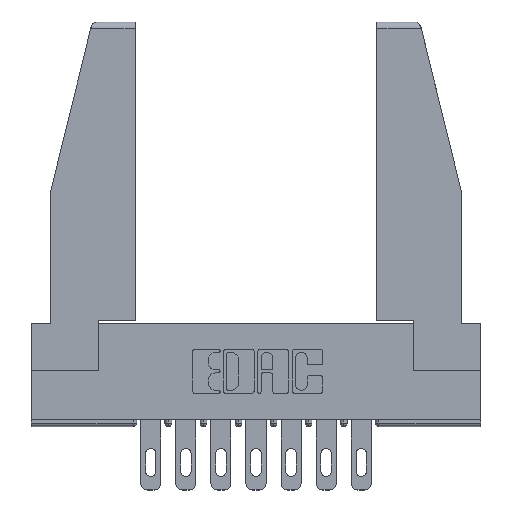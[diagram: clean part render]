
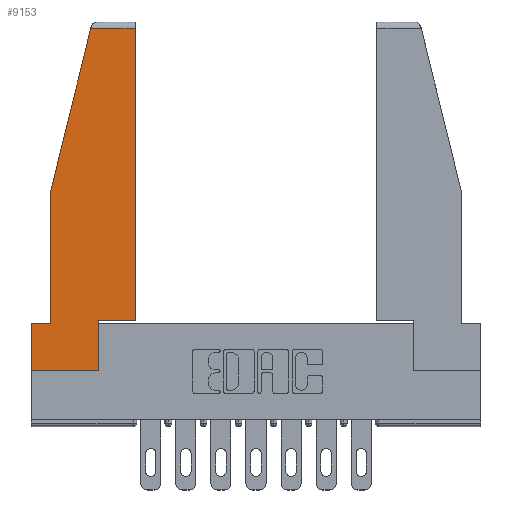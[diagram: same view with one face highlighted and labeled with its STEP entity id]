
A CAD part, top view. The second image highlights one B-rep face of the part: STEP entity #9153.
In plain terms, the highlighted planar face has unit normal (0, 0, 1).
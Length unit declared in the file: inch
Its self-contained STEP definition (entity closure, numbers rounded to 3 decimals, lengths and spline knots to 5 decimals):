
#136 = EDGE_CURVE ( 'NONE', #3867, #2991, #2911, .T. ) ;
#413 = LINE ( 'NONE', #6282, #13234 ) ;
#431 = LINE ( 'NONE', #12536, #7899 ) ;
#455 = VERTEX_POINT ( 'NONE', #8665 ) ;
#515 = DIRECTION ( 'NONE',  ( -1., 0., 0. ) ) ;
#610 = VECTOR ( 'NONE', #1914, 39.37008 ) ;
#940 = CARTESIAN_POINT ( 'NONE',  ( 0., 0.21, 0. ) ) ;
#1140 = ORIENTED_EDGE ( 'NONE', *, *, #8603, .T. ) ;
#1431 = DIRECTION ( 'NONE',  ( 0., 1., 0. ) ) ;
#1530 = ORIENTED_EDGE ( 'NONE', *, *, #7670, .T. ) ;
#1914 = DIRECTION ( 'NONE',  ( 0., 1., 0. ) ) ;
#2023 = LINE ( 'NONE', #5896, #12410 ) ;
#2159 = CARTESIAN_POINT ( 'NONE',  ( 0.086, 0.21, 0. ) ) ;
#2171 = VERTEX_POINT ( 'NONE', #7462 ) ;
#2279 = ORIENTED_EDGE ( 'NONE', *, *, #4471, .T. ) ;
#2459 = AXIS2_PLACEMENT_3D ( 'NONE', #3951, #11770, #9659 ) ;
#2619 = CARTESIAN_POINT ( 'NONE',  ( 0.297, 0., 0. ) ) ;
#2677 = CARTESIAN_POINT ( 'NONE',  ( 0.297, 0.223, 0. ) ) ;
#2857 = VERTEX_POINT ( 'NONE', #3028 ) ;
#2911 = LINE ( 'NONE', #6354, #7980 ) ;
#2991 = VERTEX_POINT ( 'NONE', #2159 ) ;
#3028 = CARTESIAN_POINT ( 'NONE',  ( 0., 0.21, 0. ) ) ;
#3124 = ORIENTED_EDGE ( 'NONE', *, *, #5001, .T. ) ;
#3164 = ORIENTED_EDGE ( 'NONE', *, *, #13414, .T. ) ;
#3232 = LINE ( 'NONE', #5779, #13629 ) ;
#3373 = CARTESIAN_POINT ( 'NONE',  ( 0.461, 1.52, 0. ) ) ;
#3582 = VERTEX_POINT ( 'NONE', #2677 ) ;
#3867 = VERTEX_POINT ( 'NONE', #7678 ) ;
#3951 = CARTESIAN_POINT ( 'NONE',  ( 0., 0., 0. ) ) ;
#4002 = CARTESIAN_POINT ( 'NONE',  ( 0.461, 0.223, 0. ) ) ;
#4132 = EDGE_LOOP ( 'NONE', ( #1140, #3124, #1530, #4251, #3164, #4920, #13564, #2279, #6168 ) ) ;
#4251 = ORIENTED_EDGE ( 'NONE', *, *, #136, .T. ) ;
#4471 = EDGE_CURVE ( 'NONE', #11924, #3582, #9983, .T. ) ;
#4920 = ORIENTED_EDGE ( 'NONE', *, *, #8428, .T. ) ;
#4953 = CARTESIAN_POINT ( 'NONE',  ( 0., 1.52, 0. ) ) ;
#5001 = EDGE_CURVE ( 'NONE', #6144, #9049, #10142, .T. ) ;
#5779 = CARTESIAN_POINT ( 'NONE',  ( 0.271, 1.55, 0. ) ) ;
#5896 = CARTESIAN_POINT ( 'NONE',  ( 0., 0.21, 0. ) ) ;
#6144 = VERTEX_POINT ( 'NONE', #3373 ) ;
#6168 = ORIENTED_EDGE ( 'NONE', *, *, #6552, .T. ) ;
#6282 = CARTESIAN_POINT ( 'NONE',  ( 0.297, 0.223, 0. ) ) ;
#6354 = CARTESIAN_POINT ( 'NONE',  ( 0.086, 0.8, 0. ) ) ;
#6382 = DIRECTION ( 'NONE',  ( 1., 0., 0. ) ) ;
#6552 = EDGE_CURVE ( 'NONE', #3582, #2171, #413, .T. ) ;
#6693 = VECTOR ( 'NONE', #515, 39.37008 ) ;
#6982 = DIRECTION ( 'NONE',  ( 1., 0., 0. ) ) ;
#7462 = CARTESIAN_POINT ( 'NONE',  ( 0.461, 0.223, 0. ) ) ;
#7670 = EDGE_CURVE ( 'NONE', #9049, #3867, #3232, .T. ) ;
#7678 = CARTESIAN_POINT ( 'NONE',  ( 0.086, 0.8, 0. ) ) ;
#7802 = LINE ( 'NONE', #940, #13302 ) ;
#7889 = DIRECTION ( 'NONE',  ( -0.239, -0.971, 0. ) ) ;
#7899 = VECTOR ( 'NONE', #6982, 39.37008 ) ;
#7933 = CARTESIAN_POINT ( 'NONE',  ( 0.297, 0., 0. ) ) ;
#7980 = VECTOR ( 'NONE', #12883, 39.37008 ) ;
#8191 = DIRECTION ( 'NONE',  ( 0., -1., 0. ) ) ;
#8428 = EDGE_CURVE ( 'NONE', #2857, #455, #2023, .T. ) ;
#8603 = EDGE_CURVE ( 'NONE', #2171, #6144, #9972, .T. ) ;
#8665 = CARTESIAN_POINT ( 'NONE',  ( 0., 0., 0. ) ) ;
#9049 = VERTEX_POINT ( 'NONE', #9209 ) ;
#9153 = ADVANCED_FACE ( 'NONE', ( #12913 ), #9755, .T. ) ;
#9168 = EDGE_CURVE ( 'NONE', #455, #11924, #431, .T. ) ;
#9209 = CARTESIAN_POINT ( 'NONE',  ( 0.2636, 1.52, 0. ) ) ;
#9659 = DIRECTION ( 'NONE',  ( 1., 0., 0. ) ) ;
#9755 = PLANE ( 'NONE',  #2459 ) ;
#9972 = LINE ( 'NONE', #4002, #610 ) ;
#9983 = LINE ( 'NONE', #7933, #11360 ) ;
#10142 = LINE ( 'NONE', #4953, #6693 ) ;
#10735 = DIRECTION ( 'NONE',  ( -1., 0., 0. ) ) ;
#11360 = VECTOR ( 'NONE', #1431, 39.37008 ) ;
#11770 = DIRECTION ( 'NONE',  ( 0., 0., 1. ) ) ;
#11924 = VERTEX_POINT ( 'NONE', #2619 ) ;
#12410 = VECTOR ( 'NONE', #8191, 39.37008 ) ;
#12536 = CARTESIAN_POINT ( 'NONE',  ( 0., 0., 0. ) ) ;
#12883 = DIRECTION ( 'NONE',  ( 0., -1., 0. ) ) ;
#12913 = FACE_OUTER_BOUND ( 'NONE', #4132, .T. ) ;
#13234 = VECTOR ( 'NONE', #6382, 39.37008 ) ;
#13302 = VECTOR ( 'NONE', #10735, 39.37008 ) ;
#13414 = EDGE_CURVE ( 'NONE', #2991, #2857, #7802, .T. ) ;
#13564 = ORIENTED_EDGE ( 'NONE', *, *, #9168, .T. ) ;
#13629 = VECTOR ( 'NONE', #7889, 39.37008 ) ;
